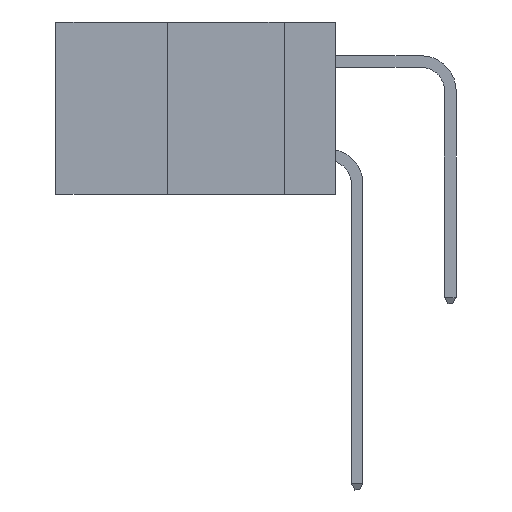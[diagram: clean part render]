
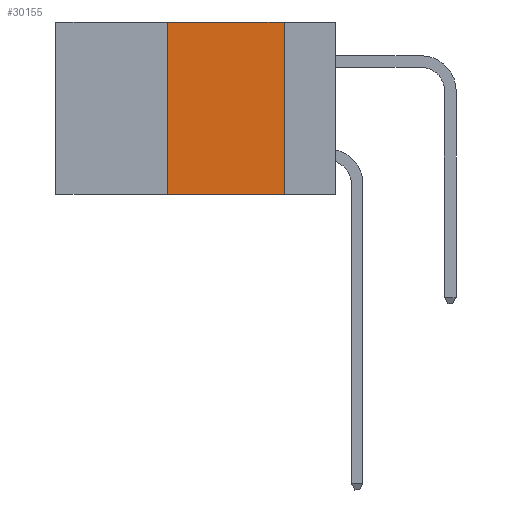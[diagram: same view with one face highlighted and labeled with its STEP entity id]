
A CAD part, left-side view. The second image highlights one B-rep face of the part: STEP entity #30155.
In plain terms, the highlighted planar face has unit normal (-1, 0, 0).
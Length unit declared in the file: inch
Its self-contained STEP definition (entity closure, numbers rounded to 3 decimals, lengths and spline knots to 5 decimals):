
#735 = EDGE_CURVE ( 'NONE', #26244, #12883, #4183, .T. ) ;
#1185 = LINE ( 'NONE', #4200, #11490 ) ;
#1247 = ORIENTED_EDGE ( 'NONE', *, *, #6850, .T. ) ;
#4183 = LINE ( 'NONE', #21167, #7829 ) ;
#4200 = CARTESIAN_POINT ( 'NONE',  ( 0., 0.6, -0.37 ) ) ;
#4942 = PLANE ( 'NONE',  #26805 ) ;
#6850 = EDGE_CURVE ( 'NONE', #27484, #14781, #1185, .T. ) ;
#7829 = VECTOR ( 'NONE', #29007, 39.37008 ) ;
#8901 = EDGE_CURVE ( 'NONE', #27484, #26244, #25750, .T. ) ;
#9984 = DIRECTION ( 'NONE',  ( 1., 0., 0. ) ) ;
#11490 = VECTOR ( 'NONE', #24972, 39.37008 ) ;
#11583 = VECTOR ( 'NONE', #30008, 39.37008 ) ;
#12571 = VECTOR ( 'NONE', #18094, 39.37008 ) ;
#12883 = VERTEX_POINT ( 'NONE', #18908 ) ;
#13885 = CARTESIAN_POINT ( 'NONE',  ( 0., 0.11, -0.37 ) ) ;
#14781 = VERTEX_POINT ( 'NONE', #13885 ) ;
#17365 = LINE ( 'NONE', #22071, #11583 ) ;
#17772 = EDGE_LOOP ( 'NONE', ( #26199, #21975, #31620, #1247 ) ) ;
#17814 = DIRECTION ( 'NONE',  ( 0., 0., -1. ) ) ;
#18094 = DIRECTION ( 'NONE',  ( 0., 0., 1. ) ) ;
#18276 = CARTESIAN_POINT ( 'NONE',  ( 0., 0.6, 0. ) ) ;
#18908 = CARTESIAN_POINT ( 'NONE',  ( 0., 0.11, 0. ) ) ;
#20704 = CARTESIAN_POINT ( 'NONE',  ( 0., 0.36, 0. ) ) ;
#21167 = CARTESIAN_POINT ( 'NONE',  ( 0., 0.6, 0. ) ) ;
#21975 = ORIENTED_EDGE ( 'NONE', *, *, #735, .F. ) ;
#22071 = CARTESIAN_POINT ( 'NONE',  ( 0., 0.11, 0. ) ) ;
#22811 = FACE_OUTER_BOUND ( 'NONE', #17772, .T. ) ;
#24972 = DIRECTION ( 'NONE',  ( 0., -1., 0. ) ) ;
#25750 = LINE ( 'NONE', #26570, #12571 ) ;
#26199 = ORIENTED_EDGE ( 'NONE', *, *, #32064, .F. ) ;
#26244 = VERTEX_POINT ( 'NONE', #20704 ) ;
#26570 = CARTESIAN_POINT ( 'NONE',  ( 0., 0.36, 0. ) ) ;
#26805 = AXIS2_PLACEMENT_3D ( 'NONE', #18276, #9984, #17814 ) ;
#27484 = VERTEX_POINT ( 'NONE', #33713 ) ;
#29007 = DIRECTION ( 'NONE',  ( 0., -1., 0. ) ) ;
#30008 = DIRECTION ( 'NONE',  ( 0., 0., -1. ) ) ;
#30155 = ADVANCED_FACE ( 'NONE', ( #22811 ), #4942, .F. ) ;
#31620 = ORIENTED_EDGE ( 'NONE', *, *, #8901, .F. ) ;
#32064 = EDGE_CURVE ( 'NONE', #12883, #14781, #17365, .T. ) ;
#33713 = CARTESIAN_POINT ( 'NONE',  ( 0., 0.36, -0.37 ) ) ;
